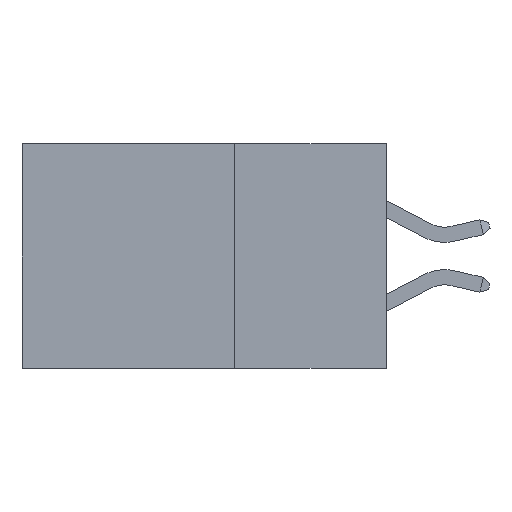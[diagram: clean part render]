
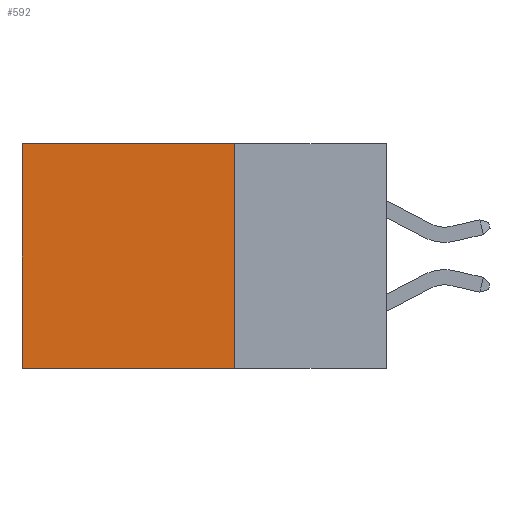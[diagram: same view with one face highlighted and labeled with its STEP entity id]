
A CAD part, left-side view. The second image highlights one B-rep face of the part: STEP entity #592.
In plain terms, the highlighted planar face has unit normal (-1, 0, 0).
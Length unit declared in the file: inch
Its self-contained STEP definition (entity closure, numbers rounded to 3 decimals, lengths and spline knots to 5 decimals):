
#592 = ADVANCED_FACE ( 'NONE', ( #23259 ), #7947, .F. ) ;
#693 = DIRECTION ( 'NONE',  ( 0., 1., 0. ) ) ;
#3172 = CARTESIAN_POINT ( 'NONE',  ( 0.2615, 0.25, 0. ) ) ;
#4655 = CARTESIAN_POINT ( 'NONE',  ( 0.2615, 0.6, -0.37 ) ) ;
#4857 = LINE ( 'NONE', #3172, #7697 ) ;
#5624 = DIRECTION ( 'NONE',  ( 0., 0., -1. ) ) ;
#6657 = AXIS2_PLACEMENT_3D ( 'NONE', #25370, #7684, #5624 ) ;
#7684 = DIRECTION ( 'NONE',  ( 1., 0., 0. ) ) ;
#7697 = VECTOR ( 'NONE', #24539, 39.37008 ) ;
#7947 = PLANE ( 'NONE',  #6657 ) ;
#8017 = EDGE_LOOP ( 'NONE', ( #8154, #12008, #22512, #21995 ) ) ;
#8154 = ORIENTED_EDGE ( 'NONE', *, *, #24895, .T. ) ;
#10364 = CARTESIAN_POINT ( 'NONE',  ( 0.2615, 0.25, 0. ) ) ;
#10671 = VECTOR ( 'NONE', #18701, 39.37008 ) ;
#10731 = VERTEX_POINT ( 'NONE', #10364 ) ;
#12008 = ORIENTED_EDGE ( 'NONE', *, *, #21014, .F. ) ;
#14377 = VECTOR ( 'NONE', #18028, 39.37008 ) ;
#16640 = VERTEX_POINT ( 'NONE', #18164 ) ;
#17292 = EDGE_CURVE ( 'NONE', #10731, #16640, #4857, .T. ) ;
#17799 = CARTESIAN_POINT ( 'NONE',  ( 0.2615, 0.6, -0.37 ) ) ;
#18028 = DIRECTION ( 'NONE',  ( 0., 0., -1. ) ) ;
#18164 = CARTESIAN_POINT ( 'NONE',  ( 0.2615, 0.6, 0. ) ) ;
#18193 = LINE ( 'NONE', #18448, #24262 ) ;
#18442 = LINE ( 'NONE', #4655, #10671 ) ;
#18448 = CARTESIAN_POINT ( 'NONE',  ( 0.2615, 0.25, -0.37 ) ) ;
#18701 = DIRECTION ( 'NONE',  ( 0., 0., -1. ) ) ;
#19377 = VERTEX_POINT ( 'NONE', #22559 ) ;
#19706 = VERTEX_POINT ( 'NONE', #17799 ) ;
#19830 = CARTESIAN_POINT ( 'NONE',  ( 0.2615, 0.25, -0.37 ) ) ;
#21014 = EDGE_CURVE ( 'NONE', #19377, #19706, #18193, .T. ) ;
#21631 = LINE ( 'NONE', #19830, #14377 ) ;
#21995 = ORIENTED_EDGE ( 'NONE', *, *, #17292, .T. ) ;
#22512 = ORIENTED_EDGE ( 'NONE', *, *, #25254, .F. ) ;
#22559 = CARTESIAN_POINT ( 'NONE',  ( 0.2615, 0.25, -0.37 ) ) ;
#23259 = FACE_OUTER_BOUND ( 'NONE', #8017, .T. ) ;
#24262 = VECTOR ( 'NONE', #693, 39.37008 ) ;
#24539 = DIRECTION ( 'NONE',  ( 0., 1., 0. ) ) ;
#24895 = EDGE_CURVE ( 'NONE', #16640, #19706, #18442, .T. ) ;
#25254 = EDGE_CURVE ( 'NONE', #10731, #19377, #21631, .T. ) ;
#25370 = CARTESIAN_POINT ( 'NONE',  ( 0.2615, 0.25, -0.37 ) ) ;
